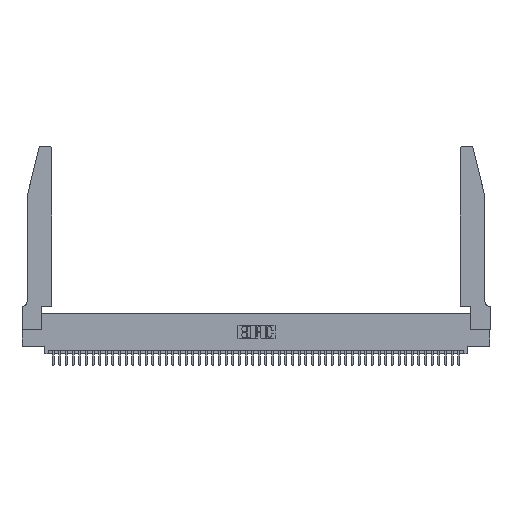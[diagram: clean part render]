
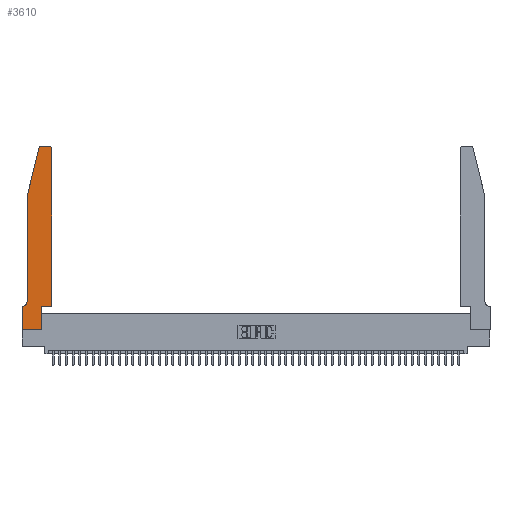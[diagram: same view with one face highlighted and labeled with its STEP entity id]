
A CAD part, top view. The second image highlights one B-rep face of the part: STEP entity #3610.
In plain terms, the highlighted planar face has unit normal (0, 0, 1).
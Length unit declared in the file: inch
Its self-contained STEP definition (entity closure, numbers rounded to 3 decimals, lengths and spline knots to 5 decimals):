
#110 = EDGE_CURVE ( 'NONE', #38058, #30023, #5489, .T. ) ;
#325 = DIRECTION ( 'NONE',  ( -1., 0., 0. ) ) ;
#637 = VERTEX_POINT ( 'NONE', #48106 ) ;
#830 = AXIS2_PLACEMENT_3D ( 'NONE', #38362, #14856, #42311 ) ;
#1076 = CARTESIAN_POINT ( 'NONE',  ( 0.2605, 2.75, 0.37 ) ) ;
#1100 = LINE ( 'NONE', #1076, #20817 ) ;
#1444 = VERTEX_POINT ( 'NONE', #17179 ) ;
#1541 = EDGE_CURVE ( 'NONE', #1444, #36942, #15822, .T. ) ;
#1627 = DIRECTION ( 'NONE',  ( 1., 0., 0. ) ) ;
#1656 = DIRECTION ( 'NONE',  ( 0., 0., -1. ) ) ;
#2837 = CARTESIAN_POINT ( 'NONE',  ( 0., 0.35, 0.37 ) ) ;
#3535 = CARTESIAN_POINT ( 'NONE',  ( 0.284, 2.72, 0.37 ) ) ;
#3610 = ADVANCED_FACE ( 'NONE', ( #3688 ), #49887, .T. ) ;
#3688 = FACE_OUTER_BOUND ( 'NONE', #42503, .T. ) ;
#3716 = CARTESIAN_POINT ( 'NONE',  ( 0.2865, 0., 0.37 ) ) ;
#3856 = EDGE_CURVE ( 'NONE', #44524, #19207, #42416, .T. ) ;
#4228 = VECTOR ( 'NONE', #22757, 39.37008 ) ;
#4478 = CARTESIAN_POINT ( 'NONE',  ( 0.0755, 2., 0.37 ) ) ;
#4590 = ORIENTED_EDGE ( 'NONE', *, *, #36199, .T. ) ;
#5252 = CARTESIAN_POINT ( 'NONE',  ( 0.0755, 2., 0.37 ) ) ;
#5489 = LINE ( 'NONE', #20876, #35600 ) ;
#6353 = ORIENTED_EDGE ( 'NONE', *, *, #36053, .T. ) ;
#6836 = DIRECTION ( 'NONE',  ( 0., 0., 1. ) ) ;
#6869 = AXIS2_PLACEMENT_3D ( 'NONE', #25215, #1656, #29206 ) ;
#7545 = DIRECTION ( 'NONE',  ( 1., 0., 0. ) ) ;
#7667 = EDGE_CURVE ( 'NONE', #15356, #37558, #16206, .T. ) ;
#8479 = DIRECTION ( 'NONE',  ( 0., -1., 0. ) ) ;
#9568 = ORIENTED_EDGE ( 'NONE', *, *, #1541, .T. ) ;
#10077 = VERTEX_POINT ( 'NONE', #28263 ) ;
#11077 = VECTOR ( 'NONE', #325, 39.37008 ) ;
#11862 = VERTEX_POINT ( 'NONE', #39123 ) ;
#11974 = VERTEX_POINT ( 'NONE', #31729 ) ;
#12280 = CARTESIAN_POINT ( 'NONE',  ( 0.4505, 0.35, 0.37 ) ) ;
#14504 = CARTESIAN_POINT ( 'NONE',  ( 0.0055, 0.35, 0.37 ) ) ;
#14856 = DIRECTION ( 'NONE',  ( 0., 0., 1. ) ) ;
#15356 = VERTEX_POINT ( 'NONE', #22817 ) ;
#15431 = CIRCLE ( 'NONE', #830, 0.03 ) ;
#15457 = EDGE_CURVE ( 'NONE', #30023, #11862, #50589, .T. ) ;
#15822 = LINE ( 'NONE', #21769, #28697 ) ;
#16206 = LINE ( 'NONE', #48721, #46278 ) ;
#16902 = CIRCLE ( 'NONE', #6869, 0.07 ) ;
#16977 = DIRECTION ( 'NONE',  ( -1., 0., 0. ) ) ;
#17179 = CARTESIAN_POINT ( 'NONE',  ( 0., 0., 0.37 ) ) ;
#18049 = EDGE_CURVE ( 'NONE', #10077, #637, #15431, .T. ) ;
#19207 = VERTEX_POINT ( 'NONE', #32530 ) ;
#19965 = AXIS2_PLACEMENT_3D ( 'NONE', #3535, #31060, #7545 ) ;
#20016 = CARTESIAN_POINT ( 'NONE',  ( 0.0755, 0.35, 0.37 ) ) ;
#20270 = DIRECTION ( 'NONE',  ( 0., 1., 0. ) ) ;
#20817 = VECTOR ( 'NONE', #16977, 39.37008 ) ;
#20876 = CARTESIAN_POINT ( 'NONE',  ( 0.0755, 2., 0.37 ) ) ;
#21045 = VECTOR ( 'NONE', #27874, 39.37008 ) ;
#21687 = ORIENTED_EDGE ( 'NONE', *, *, #110, .T. ) ;
#21769 = CARTESIAN_POINT ( 'NONE',  ( 0., 0., 0.37 ) ) ;
#22757 = DIRECTION ( 'NONE',  ( 0., -1., 0. ) ) ;
#22817 = CARTESIAN_POINT ( 'NONE',  ( 0.2865, 0.35, 0.37 ) ) ;
#24287 = ORIENTED_EDGE ( 'NONE', *, *, #31947, .T. ) ;
#24813 = DIRECTION ( 'NONE',  ( -0.239, -0.971, 0. ) ) ;
#25215 = CARTESIAN_POINT ( 'NONE',  ( 0.0055, 0.42, 0.37 ) ) ;
#26623 = ORIENTED_EDGE ( 'NONE', *, *, #49621, .T. ) ;
#27190 = CARTESIAN_POINT ( 'NONE',  ( 0.4505, 0.35, 0.37 ) ) ;
#27873 = ORIENTED_EDGE ( 'NONE', *, *, #3856, .T. ) ;
#27874 = DIRECTION ( 'NONE',  ( 0., 1., 0. ) ) ;
#28263 = CARTESIAN_POINT ( 'NONE',  ( 0.4505, 2.72, 0.37 ) ) ;
#28697 = VECTOR ( 'NONE', #49237, 39.37008 ) ;
#29206 = DIRECTION ( 'NONE',  ( -1., 0., 0. ) ) ;
#30023 = VERTEX_POINT ( 'NONE', #5252 ) ;
#31060 = DIRECTION ( 'NONE',  ( 0., 0., 1. ) ) ;
#31520 = LINE ( 'NONE', #12280, #21045 ) ;
#31729 = CARTESIAN_POINT ( 'NONE',  ( 0.284, 2.75, 0.37 ) ) ;
#31901 = LINE ( 'NONE', #47732, #33130 ) ;
#31947 = EDGE_CURVE ( 'NONE', #37558, #10077, #31520, .T. ) ;
#32530 = CARTESIAN_POINT ( 'NONE',  ( 0., 0.35, 0.37 ) ) ;
#33130 = VECTOR ( 'NONE', #20270, 39.37008 ) ;
#34310 = DIRECTION ( 'NONE',  ( 1., 0., 0. ) ) ;
#34378 = CARTESIAN_POINT ( 'NONE',  ( 0.25487, 2.72718, 0.37 ) ) ;
#34801 = ORIENTED_EDGE ( 'NONE', *, *, #18049, .T. ) ;
#35593 = LINE ( 'NONE', #50241, #4228 ) ;
#35600 = VECTOR ( 'NONE', #24813, 39.37008 ) ;
#36053 = EDGE_CURVE ( 'NONE', #637, #11974, #1100, .T. ) ;
#36199 = EDGE_CURVE ( 'NONE', #19207, #1444, #35593, .T. ) ;
#36942 = VERTEX_POINT ( 'NONE', #3716 ) ;
#37558 = VERTEX_POINT ( 'NONE', #27190 ) ;
#37822 = ORIENTED_EDGE ( 'NONE', *, *, #44870, .T. ) ;
#38058 = VERTEX_POINT ( 'NONE', #34378 ) ;
#38362 = CARTESIAN_POINT ( 'NONE',  ( 0.4205, 2.72, 0.37 ) ) ;
#38841 = EDGE_CURVE ( 'NONE', #11974, #38058, #40944, .T. ) ;
#39123 = CARTESIAN_POINT ( 'NONE',  ( 0.0755, 0.42, 0.37 ) ) ;
#40192 = VECTOR ( 'NONE', #8479, 39.37008 ) ;
#40944 = CIRCLE ( 'NONE', #19965, 0.03 ) ;
#42311 = DIRECTION ( 'NONE',  ( 1., 0., 0. ) ) ;
#42416 = LINE ( 'NONE', #20016, #11077 ) ;
#42503 = EDGE_LOOP ( 'NONE', ( #6353, #48086, #21687, #42626, #26623, #27873, #4590, #9568, #37822, #50698, #24287, #34801 ) ) ;
#42626 = ORIENTED_EDGE ( 'NONE', *, *, #15457, .T. ) ;
#43918 = AXIS2_PLACEMENT_3D ( 'NONE', #2837, #6836, #34310 ) ;
#44524 = VERTEX_POINT ( 'NONE', #14504 ) ;
#44870 = EDGE_CURVE ( 'NONE', #36942, #15356, #31901, .T. ) ;
#46278 = VECTOR ( 'NONE', #1627, 39.37008 ) ;
#47732 = CARTESIAN_POINT ( 'NONE',  ( 0.2865, 0.35, 0.37 ) ) ;
#48086 = ORIENTED_EDGE ( 'NONE', *, *, #38841, .T. ) ;
#48106 = CARTESIAN_POINT ( 'NONE',  ( 0.4205, 2.75, 0.37 ) ) ;
#48721 = CARTESIAN_POINT ( 'NONE',  ( 0.4505, 0.35, 0.37 ) ) ;
#49237 = DIRECTION ( 'NONE',  ( 1., 0., 0. ) ) ;
#49621 = EDGE_CURVE ( 'NONE', #11862, #44524, #16902, .T. ) ;
#49887 = PLANE ( 'NONE',  #43918 ) ;
#50241 = CARTESIAN_POINT ( 'NONE',  ( 0., 0., 0.37 ) ) ;
#50589 = LINE ( 'NONE', #4478, #40192 ) ;
#50698 = ORIENTED_EDGE ( 'NONE', *, *, #7667, .T. ) ;
